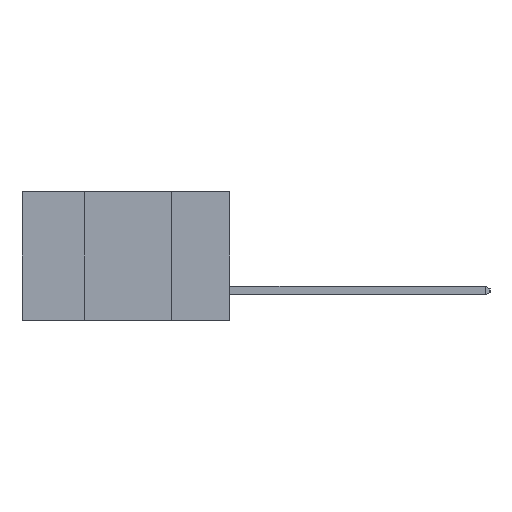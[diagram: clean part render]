
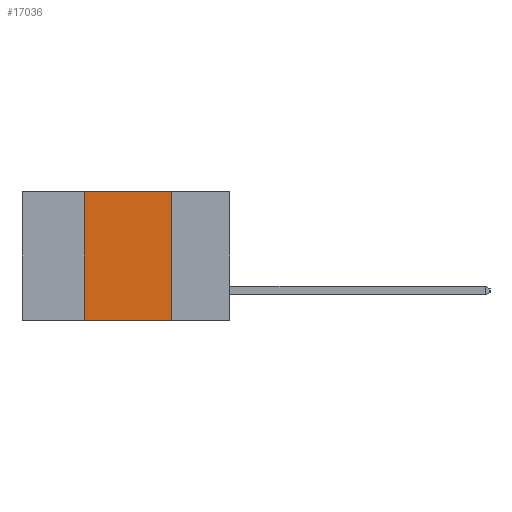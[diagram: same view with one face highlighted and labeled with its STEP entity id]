
A CAD part, left-side view. The second image highlights one B-rep face of the part: STEP entity #17036.
In plain terms, the highlighted planar face has unit normal (-1, 0, 0).
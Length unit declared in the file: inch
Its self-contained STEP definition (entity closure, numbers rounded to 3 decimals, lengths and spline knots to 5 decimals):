
#149 = DIRECTION ( 'NONE',  ( 0., -1., 0. ) ) ;
#297 = CARTESIAN_POINT ( 'NONE',  ( 0., 0.6, -0.37 ) ) ;
#932 = DIRECTION ( 'NONE',  ( 0., 0., 1. ) ) ;
#1120 = ORIENTED_EDGE ( 'NONE', *, *, #19993, .F. ) ;
#1331 = PLANE ( 'NONE',  #12190 ) ;
#1829 = VERTEX_POINT ( 'NONE', #10387 ) ;
#1918 = LINE ( 'NONE', #14663, #18626 ) ;
#3172 = LINE ( 'NONE', #14065, #15713 ) ;
#3715 = ORIENTED_EDGE ( 'NONE', *, *, #17151, .F. ) ;
#4527 = EDGE_CURVE ( 'NONE', #8089, #1829, #18656, .T. ) ;
#4599 = CARTESIAN_POINT ( 'NONE',  ( 0., 0.6, 0. ) ) ;
#4954 = DIRECTION ( 'NONE',  ( 0., 0., -1. ) ) ;
#5491 = ORIENTED_EDGE ( 'NONE', *, *, #20221, .F. ) ;
#5572 = CARTESIAN_POINT ( 'NONE',  ( 0., 0.42, -0.37 ) ) ;
#6119 = VERTEX_POINT ( 'NONE', #18453 ) ;
#6258 = DIRECTION ( 'NONE',  ( 0., 0., -1. ) ) ;
#6637 = VERTEX_POINT ( 'NONE', #8243 ) ;
#8089 = VERTEX_POINT ( 'NONE', #5572 ) ;
#8243 = CARTESIAN_POINT ( 'NONE',  ( 0., 0.42, 0. ) ) ;
#10066 = ORIENTED_EDGE ( 'NONE', *, *, #4527, .T. ) ;
#10387 = CARTESIAN_POINT ( 'NONE',  ( 0., 0.17, -0.37 ) ) ;
#11837 = LINE ( 'NONE', #14787, #20177 ) ;
#12190 = AXIS2_PLACEMENT_3D ( 'NONE', #4599, #16034, #6258 ) ;
#14065 = CARTESIAN_POINT ( 'NONE',  ( 0., 0.42, -0.37 ) ) ;
#14525 = VECTOR ( 'NONE', #149, 39.37008 ) ;
#14663 = CARTESIAN_POINT ( 'NONE',  ( 0., 0.6, 0. ) ) ;
#14787 = CARTESIAN_POINT ( 'NONE',  ( 0., 0.17, -0.37 ) ) ;
#15713 = VECTOR ( 'NONE', #932, 39.37008 ) ;
#16034 = DIRECTION ( 'NONE',  ( 1., 0., 0. ) ) ;
#16245 = DIRECTION ( 'NONE',  ( 0., -1., 0. ) ) ;
#17036 = ADVANCED_FACE ( 'NONE', ( #19461 ), #1331, .F. ) ;
#17151 = EDGE_CURVE ( 'NONE', #6119, #1829, #11837, .T. ) ;
#18453 = CARTESIAN_POINT ( 'NONE',  ( 0., 0.17, 0. ) ) ;
#18626 = VECTOR ( 'NONE', #16245, 39.37008 ) ;
#18656 = LINE ( 'NONE', #297, #14525 ) ;
#18713 = EDGE_LOOP ( 'NONE', ( #3715, #5491, #1120, #10066 ) ) ;
#19461 = FACE_OUTER_BOUND ( 'NONE', #18713, .T. ) ;
#19993 = EDGE_CURVE ( 'NONE', #8089, #6637, #3172, .T. ) ;
#20177 = VECTOR ( 'NONE', #4954, 39.37008 ) ;
#20221 = EDGE_CURVE ( 'NONE', #6637, #6119, #1918, .T. ) ;
